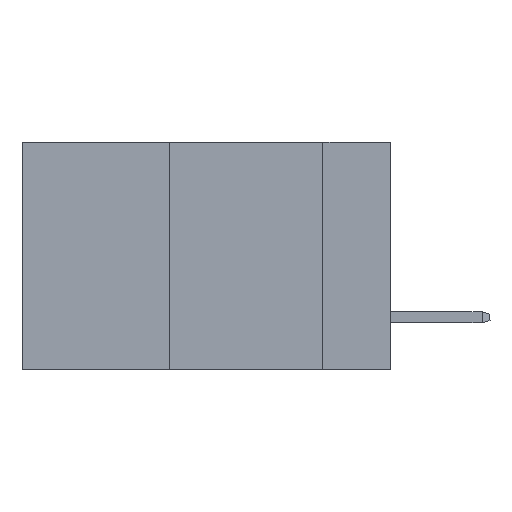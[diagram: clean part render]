
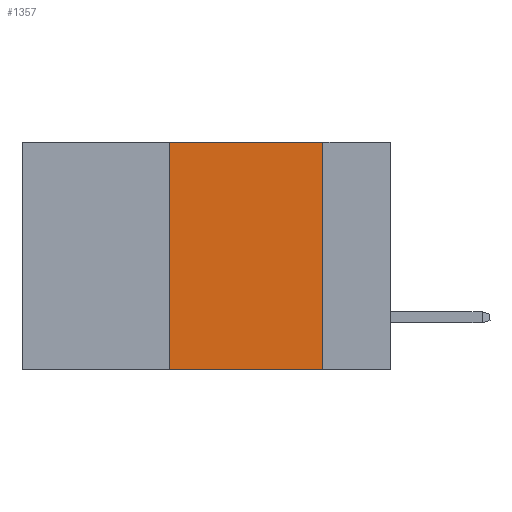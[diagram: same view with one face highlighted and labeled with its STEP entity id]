
A CAD part, left-side view. The second image highlights one B-rep face of the part: STEP entity #1357.
In plain terms, the highlighted planar face has unit normal (-1, 0, 0).
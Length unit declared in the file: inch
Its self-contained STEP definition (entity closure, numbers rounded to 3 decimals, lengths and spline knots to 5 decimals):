
#17 = ORIENTED_EDGE ( 'NONE', *, *, #6129, .T. ) ;
#1147 = VERTEX_POINT ( 'NONE', #10731 ) ;
#1224 = EDGE_CURVE ( 'NONE', #23721, #1147, #5061, .T. ) ;
#1357 = ADVANCED_FACE ( 'NONE', ( #6538 ), #17402, .F. ) ;
#5061 = LINE ( 'NONE', #21322, #20380 ) ;
#5078 = EDGE_LOOP ( 'NONE', ( #6295, #17778, #5185, #17 ) ) ;
#5185 = ORIENTED_EDGE ( 'NONE', *, *, #10927, .F. ) ;
#6129 = EDGE_CURVE ( 'NONE', #19266, #1147, #16086, .T. ) ;
#6225 = CARTESIAN_POINT ( 'NONE',  ( 0., 0.36, 0. ) ) ;
#6295 = ORIENTED_EDGE ( 'NONE', *, *, #1224, .F. ) ;
#6321 = VECTOR ( 'NONE', #13543, 39.37008 ) ;
#6538 = FACE_OUTER_BOUND ( 'NONE', #5078, .T. ) ;
#10731 = CARTESIAN_POINT ( 'NONE',  ( 0., 0.11, -0.37 ) ) ;
#10927 = EDGE_CURVE ( 'NONE', #19266, #16652, #13254, .T. ) ;
#11319 = CARTESIAN_POINT ( 'NONE',  ( 0., 0.6, 0. ) ) ;
#11356 = DIRECTION ( 'NONE',  ( 0., 0., -1. ) ) ;
#11705 = CARTESIAN_POINT ( 'NONE',  ( 0., 0.6, -0.37 ) ) ;
#12380 = DIRECTION ( 'NONE',  ( 0., 0., 1. ) ) ;
#13204 = CARTESIAN_POINT ( 'NONE',  ( 0., 0.11, 0. ) ) ;
#13254 = LINE ( 'NONE', #17849, #22585 ) ;
#13543 = DIRECTION ( 'NONE',  ( 0., -1., 0. ) ) ;
#16086 = LINE ( 'NONE', #11705, #6321 ) ;
#16652 = VERTEX_POINT ( 'NONE', #6225 ) ;
#17402 = PLANE ( 'NONE',  #24155 ) ;
#17778 = ORIENTED_EDGE ( 'NONE', *, *, #23048, .F. ) ;
#17849 = CARTESIAN_POINT ( 'NONE',  ( 0., 0.36, 0. ) ) ;
#18081 = DIRECTION ( 'NONE',  ( 0., 0., -1. ) ) ;
#18176 = CARTESIAN_POINT ( 'NONE',  ( 0., 0.6, 0. ) ) ;
#18233 = DIRECTION ( 'NONE',  ( 1., 0., 0. ) ) ;
#18821 = CARTESIAN_POINT ( 'NONE',  ( 0., 0.36, -0.37 ) ) ;
#19097 = VECTOR ( 'NONE', #20535, 39.37008 ) ;
#19266 = VERTEX_POINT ( 'NONE', #18821 ) ;
#19696 = LINE ( 'NONE', #11319, #19097 ) ;
#20380 = VECTOR ( 'NONE', #11356, 39.37008 ) ;
#20535 = DIRECTION ( 'NONE',  ( 0., -1., 0. ) ) ;
#21322 = CARTESIAN_POINT ( 'NONE',  ( 0., 0.11, 0. ) ) ;
#22585 = VECTOR ( 'NONE', #12380, 39.37008 ) ;
#23048 = EDGE_CURVE ( 'NONE', #16652, #23721, #19696, .T. ) ;
#23721 = VERTEX_POINT ( 'NONE', #13204 ) ;
#24155 = AXIS2_PLACEMENT_3D ( 'NONE', #18176, #18233, #18081 ) ;
